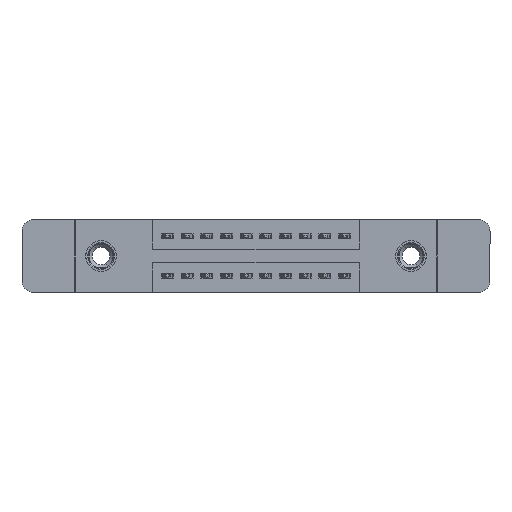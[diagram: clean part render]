
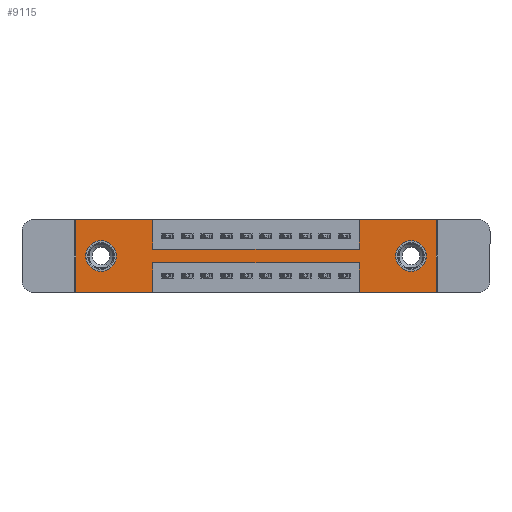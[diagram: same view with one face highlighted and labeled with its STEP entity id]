
A CAD part, front view. The second image highlights one B-rep face of the part: STEP entity #9115.
In plain terms, the highlighted planar face has unit normal (0, -1, 0).
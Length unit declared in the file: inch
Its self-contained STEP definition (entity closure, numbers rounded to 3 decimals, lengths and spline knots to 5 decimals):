
#13 = VECTOR ( 'NONE', #209, 39.37008 ) ;
#123 = AXIS2_PLACEMENT_3D ( 'NONE', #15727, #3814, #1051 ) ;
#161 = CARTESIAN_POINT ( 'NONE',  ( 0.3925, 0., -0.22 ) ) ;
#209 = DIRECTION ( 'NONE',  ( 1., 0., 0. ) ) ;
#445 = EDGE_CURVE ( 'NONE', #7660, #14005, #12660, .T. ) ;
#486 = VERTEX_POINT ( 'NONE', #5850 ) ;
#600 = CARTESIAN_POINT ( 'NONE',  ( 0.3925, 0., -0.15 ) ) ;
#739 = DIRECTION ( 'NONE',  ( 1., 0., 0. ) ) ;
#930 = EDGE_CURVE ( 'NONE', #15644, #5386, #5631, .T. ) ;
#1000 = ORIENTED_EDGE ( 'NONE', *, *, #13196, .F. ) ;
#1051 = DIRECTION ( 'NONE',  ( 0., 0., -1. ) ) ;
#1278 = VERTEX_POINT ( 'NONE', #15030 ) ;
#1295 = ORIENTED_EDGE ( 'NONE', *, *, #5012, .F. ) ;
#1632 = AXIS2_PLACEMENT_3D ( 'NONE', #6807, #6699, #6645 ) ;
#1669 = CARTESIAN_POINT ( 'NONE',  ( 1.705, 0., -0.185 ) ) ;
#1709 = DIRECTION ( 'NONE',  ( 0., 1., 0. ) ) ;
#1853 = DIRECTION ( 'NONE',  ( 0., 0., -1. ) ) ;
#1933 = VECTOR ( 'NONE', #4628, 39.37008 ) ;
#2184 = VERTEX_POINT ( 'NONE', #13845 ) ;
#2337 = VERTEX_POINT ( 'NONE', #12606 ) ;
#2400 = VERTEX_POINT ( 'NONE', #12048 ) ;
#2438 = LINE ( 'NONE', #10484, #9145 ) ;
#2769 = ORIENTED_EDGE ( 'NONE', *, *, #16015, .T. ) ;
#2861 = FACE_BOUND ( 'NONE', #10184, .T. ) ;
#2862 = DIRECTION ( 'NONE',  ( 0., 0., 1. ) ) ;
#2929 = CARTESIAN_POINT ( 'NONE',  ( 1.4425, 0., -0.15 ) ) ;
#2950 = AXIS2_PLACEMENT_3D ( 'NONE', #6878, #16074, #8176 ) ;
#2987 = CARTESIAN_POINT ( 'NONE',  ( 0.3925, 0., -0.15 ) ) ;
#3094 = DIRECTION ( 'NONE',  ( 0., 0., -1. ) ) ;
#3218 = CARTESIAN_POINT ( 'NONE',  ( 1.835, 0., 0. ) ) ;
#3320 = FACE_OUTER_BOUND ( 'NONE', #7294, .T. ) ;
#3458 = ORIENTED_EDGE ( 'NONE', *, *, #12903, .F. ) ;
#3580 = ORIENTED_EDGE ( 'NONE', *, *, #930, .F. ) ;
#3588 = VERTEX_POINT ( 'NONE', #600 ) ;
#3814 = DIRECTION ( 'NONE',  ( 0., -1., 0. ) ) ;
#4146 = CARTESIAN_POINT ( 'NONE',  ( 1.835, 0., -0.37 ) ) ;
#4192 = VERTEX_POINT ( 'NONE', #161 ) ;
#4301 = ORIENTED_EDGE ( 'NONE', *, *, #7669, .F. ) ;
#4340 = VECTOR ( 'NONE', #1853, 39.37008 ) ;
#4453 = LINE ( 'NONE', #10782, #14572 ) ;
#4628 = DIRECTION ( 'NONE',  ( 0., 0., 1. ) ) ;
#4712 = CARTESIAN_POINT ( 'NONE',  ( 0.13, 0., -0.263 ) ) ;
#4913 = VERTEX_POINT ( 'NONE', #5336 ) ;
#5012 = EDGE_CURVE ( 'NONE', #4913, #2400, #4453, .T. ) ;
#5124 = EDGE_CURVE ( 'NONE', #15322, #15644, #16832, .T. ) ;
#5336 = CARTESIAN_POINT ( 'NONE',  ( 0.3925, 0., -0.37 ) ) ;
#5357 = EDGE_CURVE ( 'NONE', #486, #2184, #17026, .T. ) ;
#5386 = VERTEX_POINT ( 'NONE', #16872 ) ;
#5626 = DIRECTION ( 'NONE',  ( -1., 0., 0. ) ) ;
#5631 = LINE ( 'NONE', #12581, #1933 ) ;
#5754 = ORIENTED_EDGE ( 'NONE', *, *, #445, .T. ) ;
#5850 = CARTESIAN_POINT ( 'NONE',  ( 0., 0., 0. ) ) ;
#6086 = EDGE_LOOP ( 'NONE', ( #5754, #2769 ) ) ;
#6340 = CARTESIAN_POINT ( 'NONE',  ( 1.4425, 0., -0.37 ) ) ;
#6413 = CARTESIAN_POINT ( 'NONE',  ( 0.3925, 0., 0. ) ) ;
#6570 = LINE ( 'NONE', #9515, #13158 ) ;
#6610 = EDGE_CURVE ( 'NONE', #16706, #1278, #6702, .T. ) ;
#6632 = CIRCLE ( 'NONE', #7300, 0.078 ) ;
#6645 = DIRECTION ( 'NONE',  ( 0., 0., -1. ) ) ;
#6699 = DIRECTION ( 'NONE',  ( 0., 1., 0. ) ) ;
#6702 = CIRCLE ( 'NONE', #2950, 0.078 ) ;
#6749 = VECTOR ( 'NONE', #11140, 39.37008 ) ;
#6807 = CARTESIAN_POINT ( 'NONE',  ( 1.705, 0., -0.185 ) ) ;
#6878 = CARTESIAN_POINT ( 'NONE',  ( 0.13, 0., -0.185 ) ) ;
#6906 = FACE_BOUND ( 'NONE', #6086, .T. ) ;
#6942 = VECTOR ( 'NONE', #739, 39.37008 ) ;
#7163 = DIRECTION ( 'NONE',  ( 0., 0., 1. ) ) ;
#7179 = VECTOR ( 'NONE', #11711, 39.37008 ) ;
#7207 = DIRECTION ( 'NONE',  ( -1., 0., 0. ) ) ;
#7294 = EDGE_LOOP ( 'NONE', ( #14495, #4301, #3580, #9501, #14938, #16861, #14132, #11912, #3458, #14193, #1000, #1295 ) ) ;
#7300 = AXIS2_PLACEMENT_3D ( 'NONE', #9783, #1709, #11127 ) ;
#7660 = VERTEX_POINT ( 'NONE', #16363 ) ;
#7669 = EDGE_CURVE ( 'NONE', #5386, #4192, #14162, .T. ) ;
#7963 = EDGE_CURVE ( 'NONE', #16640, #2337, #2438, .T. ) ;
#8107 = VERTEX_POINT ( 'NONE', #2929 ) ;
#8176 = DIRECTION ( 'NONE',  ( 0., 0., 1. ) ) ;
#8341 = LINE ( 'NONE', #16380, #14953 ) ;
#8790 = EDGE_CURVE ( 'NONE', #8107, #16640, #8341, .T. ) ;
#9115 = ADVANCED_FACE ( 'NONE', ( #6906, #2861, #3320 ), #17049, .T. ) ;
#9145 = VECTOR ( 'NONE', #13142, 39.37008 ) ;
#9501 = ORIENTED_EDGE ( 'NONE', *, *, #5124, .F. ) ;
#9515 = CARTESIAN_POINT ( 'NONE',  ( 0., 0., 0. ) ) ;
#9783 = CARTESIAN_POINT ( 'NONE',  ( 0.13, 0., -0.185 ) ) ;
#9795 = CARTESIAN_POINT ( 'NONE',  ( 0., 0., -0.37 ) ) ;
#9848 = CARTESIAN_POINT ( 'NONE',  ( 0.3925, 0., -0.22 ) ) ;
#10055 = VECTOR ( 'NONE', #11315, 39.37008 ) ;
#10184 = EDGE_LOOP ( 'NONE', ( #16778, #16901 ) ) ;
#10484 = CARTESIAN_POINT ( 'NONE',  ( 0., 0., 0. ) ) ;
#10724 = EDGE_CURVE ( 'NONE', #2337, #15322, #11814, .T. ) ;
#10782 = CARTESIAN_POINT ( 'NONE',  ( 0., 0., -0.37 ) ) ;
#11085 = DIRECTION ( 'NONE',  ( 0., 1., 0. ) ) ;
#11127 = DIRECTION ( 'NONE',  ( 0., 0., 1. ) ) ;
#11140 = DIRECTION ( 'NONE',  ( -1., 0., 0. ) ) ;
#11315 = DIRECTION ( 'NONE',  ( 0., 0., -1. ) ) ;
#11339 = EDGE_CURVE ( 'NONE', #1278, #16706, #6632, .T. ) ;
#11388 = CARTESIAN_POINT ( 'NONE',  ( 1.705, 0., -0.263 ) ) ;
#11711 = DIRECTION ( 'NONE',  ( 0., 0., -1. ) ) ;
#11814 = LINE ( 'NONE', #3218, #4340 ) ;
#11912 = ORIENTED_EDGE ( 'NONE', *, *, #14979, .F. ) ;
#12048 = CARTESIAN_POINT ( 'NONE',  ( 0., 0., -0.37 ) ) ;
#12581 = CARTESIAN_POINT ( 'NONE',  ( 1.4425, 0., -0.37 ) ) ;
#12606 = CARTESIAN_POINT ( 'NONE',  ( 1.835, 0., 0. ) ) ;
#12660 = CIRCLE ( 'NONE', #1632, 0.078 ) ;
#12872 = CARTESIAN_POINT ( 'NONE',  ( 0., 0., 0. ) ) ;
#12903 = EDGE_CURVE ( 'NONE', #2184, #3588, #14600, .T. ) ;
#13142 = DIRECTION ( 'NONE',  ( 1., 0., 0. ) ) ;
#13158 = VECTOR ( 'NONE', #2862, 39.37008 ) ;
#13196 = EDGE_CURVE ( 'NONE', #2400, #486, #6570, .T. ) ;
#13562 = LINE ( 'NONE', #16591, #10055 ) ;
#13845 = CARTESIAN_POINT ( 'NONE',  ( 0.3925, 0., 0. ) ) ;
#13853 = CARTESIAN_POINT ( 'NONE',  ( 1.4425, 0., 0. ) ) ;
#14005 = VERTEX_POINT ( 'NONE', #11388 ) ;
#14132 = ORIENTED_EDGE ( 'NONE', *, *, #8790, .F. ) ;
#14162 = LINE ( 'NONE', #9848, #17198 ) ;
#14193 = ORIENTED_EDGE ( 'NONE', *, *, #5357, .F. ) ;
#14383 = LINE ( 'NONE', #2987, #13 ) ;
#14442 = AXIS2_PLACEMENT_3D ( 'NONE', #1669, #11085, #3094 ) ;
#14495 = ORIENTED_EDGE ( 'NONE', *, *, #14526, .F. ) ;
#14526 = EDGE_CURVE ( 'NONE', #4192, #4913, #13562, .T. ) ;
#14572 = VECTOR ( 'NONE', #5626, 39.37008 ) ;
#14600 = LINE ( 'NONE', #6413, #7179 ) ;
#14938 = ORIENTED_EDGE ( 'NONE', *, *, #10724, .F. ) ;
#14953 = VECTOR ( 'NONE', #7163, 39.37008 ) ;
#14979 = EDGE_CURVE ( 'NONE', #3588, #8107, #14383, .T. ) ;
#15030 = CARTESIAN_POINT ( 'NONE',  ( 0.13, 0., -0.107 ) ) ;
#15322 = VERTEX_POINT ( 'NONE', #4146 ) ;
#15644 = VERTEX_POINT ( 'NONE', #6340 ) ;
#15648 = CIRCLE ( 'NONE', #14442, 0.078 ) ;
#15727 = CARTESIAN_POINT ( 'NONE',  ( 0., 0., -0.37 ) ) ;
#16015 = EDGE_CURVE ( 'NONE', #14005, #7660, #15648, .T. ) ;
#16074 = DIRECTION ( 'NONE',  ( 0., 1., 0. ) ) ;
#16363 = CARTESIAN_POINT ( 'NONE',  ( 1.705, 0., -0.107 ) ) ;
#16380 = CARTESIAN_POINT ( 'NONE',  ( 1.4425, 0., 0. ) ) ;
#16591 = CARTESIAN_POINT ( 'NONE',  ( 0.3925, 0., -0.37 ) ) ;
#16640 = VERTEX_POINT ( 'NONE', #13853 ) ;
#16706 = VERTEX_POINT ( 'NONE', #4712 ) ;
#16778 = ORIENTED_EDGE ( 'NONE', *, *, #11339, .T. ) ;
#16832 = LINE ( 'NONE', #9795, #6749 ) ;
#16861 = ORIENTED_EDGE ( 'NONE', *, *, #7963, .F. ) ;
#16872 = CARTESIAN_POINT ( 'NONE',  ( 1.4425, 0., -0.22 ) ) ;
#16901 = ORIENTED_EDGE ( 'NONE', *, *, #6610, .T. ) ;
#17026 = LINE ( 'NONE', #12872, #6942 ) ;
#17049 = PLANE ( 'NONE',  #123 ) ;
#17198 = VECTOR ( 'NONE', #7207, 39.37008 ) ;
